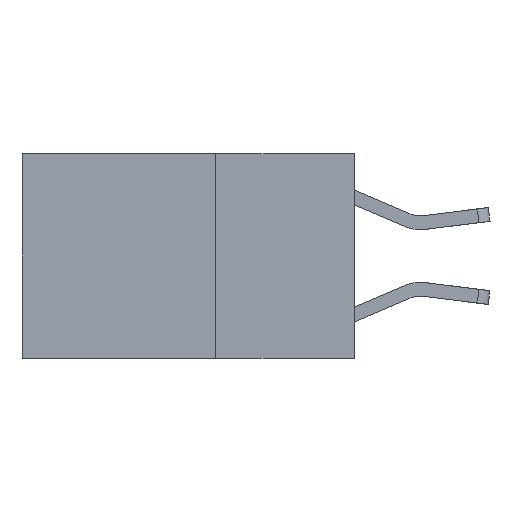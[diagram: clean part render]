
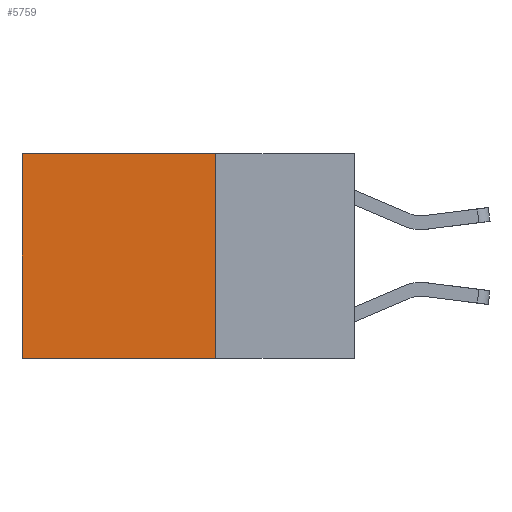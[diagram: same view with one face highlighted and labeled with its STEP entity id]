
A CAD part, left-side view. The second image highlights one B-rep face of the part: STEP entity #5759.
In plain terms, the highlighted planar face has unit normal (-1, 0, 0).
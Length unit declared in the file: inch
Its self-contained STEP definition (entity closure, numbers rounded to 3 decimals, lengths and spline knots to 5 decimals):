
#880 = EDGE_CURVE ( 'NONE', #1882, #1077, #1010, .T. ) ;
#922 = LINE ( 'NONE', #6764, #10391 ) ;
#1010 = LINE ( 'NONE', #3867, #5872 ) ;
#1077 = VERTEX_POINT ( 'NONE', #9756 ) ;
#1328 = DIRECTION ( 'NONE',  ( 0., 1., 0. ) ) ;
#1363 = FACE_OUTER_BOUND ( 'NONE', #1826, .T. ) ;
#1554 = CARTESIAN_POINT ( 'NONE',  ( 0.2625, 0.25, 0. ) ) ;
#1826 = EDGE_LOOP ( 'NONE', ( #3497, #10032, #9207, #4840 ) ) ;
#1882 = VERTEX_POINT ( 'NONE', #1554 ) ;
#2041 = LINE ( 'NONE', #10202, #10998 ) ;
#2580 = DIRECTION ( 'NONE',  ( 0., 0., -1. ) ) ;
#2919 = VECTOR ( 'NONE', #4621, 39.37008 ) ;
#3051 = EDGE_CURVE ( 'NONE', #1882, #11051, #5240, .T. ) ;
#3133 = AXIS2_PLACEMENT_3D ( 'NONE', #5498, #8140, #2580 ) ;
#3497 = ORIENTED_EDGE ( 'NONE', *, *, #4926, .T. ) ;
#3867 = CARTESIAN_POINT ( 'NONE',  ( 0.2625, 0.25, 0. ) ) ;
#4621 = DIRECTION ( 'NONE',  ( 0., 0., -1. ) ) ;
#4840 = ORIENTED_EDGE ( 'NONE', *, *, #880, .T. ) ;
#4926 = EDGE_CURVE ( 'NONE', #1077, #9641, #922, .T. ) ;
#5240 = LINE ( 'NONE', #9789, #2919 ) ;
#5498 = CARTESIAN_POINT ( 'NONE',  ( 0.2625, 0.25, 0. ) ) ;
#5759 = ADVANCED_FACE ( 'NONE', ( #1363 ), #7324, .F. ) ;
#5872 = VECTOR ( 'NONE', #6224, 39.37008 ) ;
#6224 = DIRECTION ( 'NONE',  ( 0., 1., 0. ) ) ;
#6729 = CARTESIAN_POINT ( 'NONE',  ( 0.2625, 0.6, -0.37 ) ) ;
#6764 = CARTESIAN_POINT ( 'NONE',  ( 0.2625, 0.6, 0. ) ) ;
#7324 = PLANE ( 'NONE',  #3133 ) ;
#8140 = DIRECTION ( 'NONE',  ( 1., 0., 0. ) ) ;
#8586 = CARTESIAN_POINT ( 'NONE',  ( 0.2625, 0.25, -0.37 ) ) ;
#8683 = EDGE_CURVE ( 'NONE', #11051, #9641, #2041, .T. ) ;
#9207 = ORIENTED_EDGE ( 'NONE', *, *, #3051, .F. ) ;
#9641 = VERTEX_POINT ( 'NONE', #6729 ) ;
#9756 = CARTESIAN_POINT ( 'NONE',  ( 0.2625, 0.6, 0. ) ) ;
#9789 = CARTESIAN_POINT ( 'NONE',  ( 0.2625, 0.25, 0. ) ) ;
#10032 = ORIENTED_EDGE ( 'NONE', *, *, #8683, .F. ) ;
#10202 = CARTESIAN_POINT ( 'NONE',  ( 0.2625, 0.25, -0.37 ) ) ;
#10391 = VECTOR ( 'NONE', #11392, 39.37008 ) ;
#10998 = VECTOR ( 'NONE', #1328, 39.37008 ) ;
#11051 = VERTEX_POINT ( 'NONE', #8586 ) ;
#11392 = DIRECTION ( 'NONE',  ( 0., 0., -1. ) ) ;
